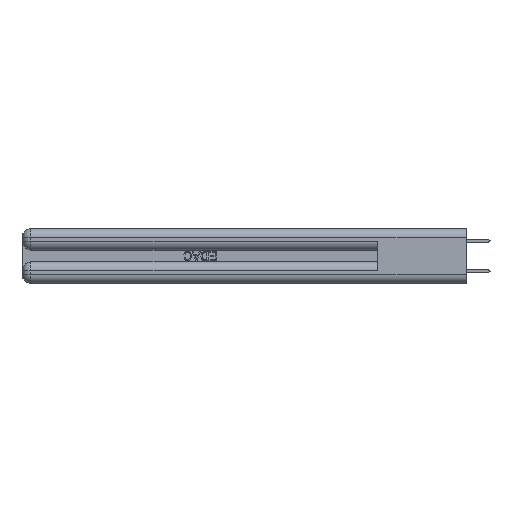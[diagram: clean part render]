
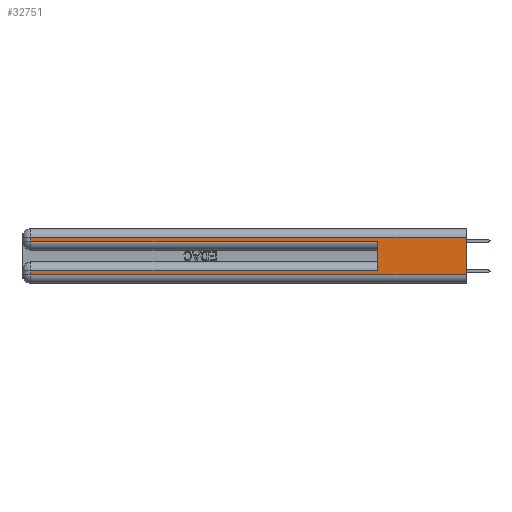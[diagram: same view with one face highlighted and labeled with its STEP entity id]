
A CAD part, left-side view. The second image highlights one B-rep face of the part: STEP entity #32751.
In plain terms, the highlighted planar face has unit normal (-1, 0, 0).
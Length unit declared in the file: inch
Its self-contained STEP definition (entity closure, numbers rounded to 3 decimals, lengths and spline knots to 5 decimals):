
#989 = EDGE_LOOP ( 'NONE', ( #11930, #40276, #12518, #15849, #35876, #27570, #43667, #37567 ) ) ;
#1695 = CARTESIAN_POINT ( 'NONE',  ( 0., 2.94, 0.06 ) ) ;
#2885 = EDGE_CURVE ( 'NONE', #3744, #15234, #21779, .T. ) ;
#3744 = VERTEX_POINT ( 'NONE', #4419 ) ;
#3902 = CARTESIAN_POINT ( 'NONE',  ( 0., 0.6, 0.285 ) ) ;
#3911 = VECTOR ( 'NONE', #12639, 39.37008 ) ;
#3965 = CARTESIAN_POINT ( 'NONE',  ( 0., 2.94, 0.31 ) ) ;
#4419 = CARTESIAN_POINT ( 'NONE',  ( 0., 0., 0.31 ) ) ;
#6106 = CARTESIAN_POINT ( 'NONE',  ( 0., 0., 0.06 ) ) ;
#6156 = VECTOR ( 'NONE', #36373, 39.37008 ) ;
#6767 = CARTESIAN_POINT ( 'NONE',  ( 0., 0., 0.37 ) ) ;
#7948 = VECTOR ( 'NONE', #33542, 39.37008 ) ;
#7974 = FACE_OUTER_BOUND ( 'NONE', #989, .T. ) ;
#9045 = CARTESIAN_POINT ( 'NONE',  ( 0., 0., 0.06 ) ) ;
#10918 = VECTOR ( 'NONE', #43583, 39.37008 ) ;
#11930 = ORIENTED_EDGE ( 'NONE', *, *, #32984, .F. ) ;
#12518 = ORIENTED_EDGE ( 'NONE', *, *, #42795, .T. ) ;
#12599 = DIRECTION ( 'NONE',  ( 0., 0., 1. ) ) ;
#12639 = DIRECTION ( 'NONE',  ( 0., -1., 0. ) ) ;
#13903 = VERTEX_POINT ( 'NONE', #45745 ) ;
#13950 = PLANE ( 'NONE',  #19221 ) ;
#14055 = VERTEX_POINT ( 'NONE', #3902 ) ;
#15083 = CARTESIAN_POINT ( 'NONE',  ( 0., 0., 0.285 ) ) ;
#15234 = VERTEX_POINT ( 'NONE', #3965 ) ;
#15630 = LINE ( 'NONE', #15083, #6156 ) ;
#15840 = CARTESIAN_POINT ( 'NONE',  ( 0., 2.94, 0.37 ) ) ;
#15849 = ORIENTED_EDGE ( 'NONE', *, *, #43934, .T. ) ;
#17442 = LINE ( 'NONE', #15840, #7948 ) ;
#17523 = DIRECTION ( 'NONE',  ( 1., 0., 0. ) ) ;
#17731 = VERTEX_POINT ( 'NONE', #36843 ) ;
#18036 = CARTESIAN_POINT ( 'NONE',  ( 0., 0., 0.085 ) ) ;
#19221 = AXIS2_PLACEMENT_3D ( 'NONE', #6767, #17523, #42383 ) ;
#20586 = EDGE_CURVE ( 'NONE', #26791, #17731, #33292, .T. ) ;
#21130 = DIRECTION ( 'NONE',  ( 0., 1., 0. ) ) ;
#21614 = DIRECTION ( 'NONE',  ( 0., 1., 0. ) ) ;
#21779 = LINE ( 'NONE', #24727, #39557 ) ;
#23959 = LINE ( 'NONE', #9045, #3911 ) ;
#24727 = CARTESIAN_POINT ( 'NONE',  ( 0., 0., 0.31 ) ) ;
#25738 = CARTESIAN_POINT ( 'NONE',  ( 0., 2.94, 0.37 ) ) ;
#25908 = CARTESIAN_POINT ( 'NONE',  ( 0., 0.6, 0.085 ) ) ;
#26346 = VECTOR ( 'NONE', #40008, 39.37008 ) ;
#26791 = VERTEX_POINT ( 'NONE', #25908 ) ;
#27570 = ORIENTED_EDGE ( 'NONE', *, *, #20586, .T. ) ;
#29330 = CARTESIAN_POINT ( 'NONE',  ( 0., 0., 0.37 ) ) ;
#30336 = CARTESIAN_POINT ( 'NONE',  ( 0., 0.6, 0.145 ) ) ;
#32751 = ADVANCED_FACE ( 'NONE', ( #7974 ), #13950, .F. ) ;
#32984 = EDGE_CURVE ( 'NONE', #3744, #37461, #45235, .T. ) ;
#33292 = LINE ( 'NONE', #18036, #41652 ) ;
#33542 = DIRECTION ( 'NONE',  ( 0., 0., -1. ) ) ;
#35765 = EDGE_CURVE ( 'NONE', #17731, #44084, #39282, .T. ) ;
#35876 = ORIENTED_EDGE ( 'NONE', *, *, #44120, .F. ) ;
#36373 = DIRECTION ( 'NONE',  ( 0., -1., 0. ) ) ;
#36843 = CARTESIAN_POINT ( 'NONE',  ( 0., 2.94, 0.085 ) ) ;
#37461 = VERTEX_POINT ( 'NONE', #6106 ) ;
#37567 = ORIENTED_EDGE ( 'NONE', *, *, #39898, .T. ) ;
#39282 = LINE ( 'NONE', #25738, #10918 ) ;
#39557 = VECTOR ( 'NONE', #21130, 39.37008 ) ;
#39898 = EDGE_CURVE ( 'NONE', #44084, #37461, #23959, .T. ) ;
#40008 = DIRECTION ( 'NONE',  ( 0., 0., -1. ) ) ;
#40276 = ORIENTED_EDGE ( 'NONE', *, *, #2885, .T. ) ;
#41652 = VECTOR ( 'NONE', #21614, 39.37008 ) ;
#42383 = DIRECTION ( 'NONE',  ( 0., 0., -1. ) ) ;
#42795 = EDGE_CURVE ( 'NONE', #15234, #13903, #17442, .T. ) ;
#43583 = DIRECTION ( 'NONE',  ( 0., 0., -1. ) ) ;
#43667 = ORIENTED_EDGE ( 'NONE', *, *, #35765, .T. ) ;
#43934 = EDGE_CURVE ( 'NONE', #13903, #14055, #15630, .T. ) ;
#44084 = VERTEX_POINT ( 'NONE', #1695 ) ;
#44120 = EDGE_CURVE ( 'NONE', #26791, #14055, #45672, .T. ) ;
#44541 = VECTOR ( 'NONE', #12599, 39.37008 ) ;
#45235 = LINE ( 'NONE', #29330, #26346 ) ;
#45672 = LINE ( 'NONE', #30336, #44541 ) ;
#45745 = CARTESIAN_POINT ( 'NONE',  ( 0., 2.94, 0.285 ) ) ;
